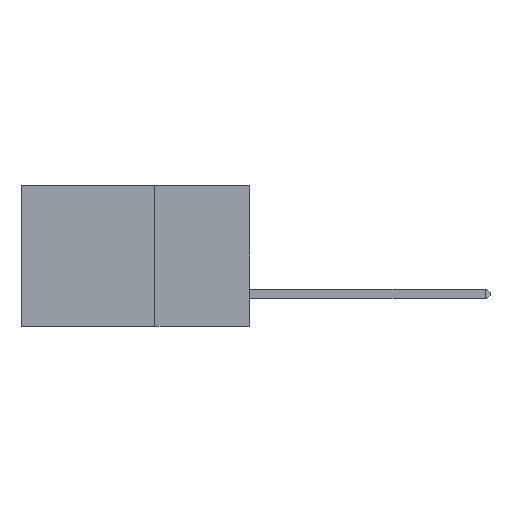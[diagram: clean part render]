
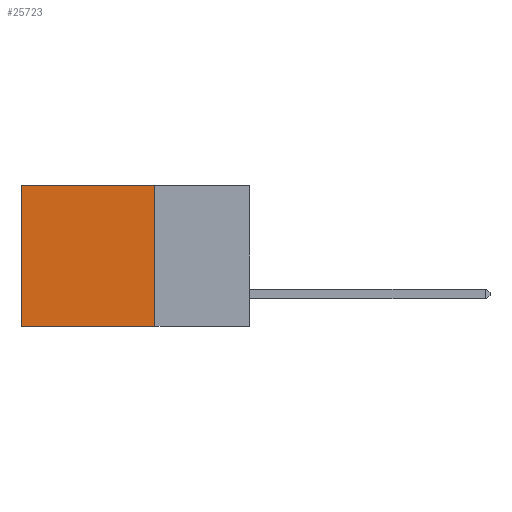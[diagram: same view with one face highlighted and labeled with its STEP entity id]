
A CAD part, left-side view. The second image highlights one B-rep face of the part: STEP entity #25723.
In plain terms, the highlighted planar face has unit normal (-1, 0, 0).
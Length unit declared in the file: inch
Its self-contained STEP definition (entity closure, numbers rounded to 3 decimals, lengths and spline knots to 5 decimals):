
#2175 = DIRECTION ( 'NONE',  ( 0., 1., 0. ) ) ;
#4576 = EDGE_CURVE ( 'NONE', #7238, #12971, #31821, .T. ) ;
#4618 = AXIS2_PLACEMENT_3D ( 'NONE', #30808, #13697, #33624 ) ;
#5003 = CARTESIAN_POINT ( 'NONE',  ( 0.2875, 0.25, -0.37 ) ) ;
#5343 = DIRECTION ( 'NONE',  ( 0., 0., -1. ) ) ;
#5471 = ORIENTED_EDGE ( 'NONE', *, *, #14323, .F. ) ;
#5676 = VECTOR ( 'NONE', #25467, 39.37008 ) ;
#6939 = LINE ( 'NONE', #13824, #34644 ) ;
#7238 = VERTEX_POINT ( 'NONE', #11531 ) ;
#8082 = CARTESIAN_POINT ( 'NONE',  ( 0.2875, 0.6, -0.37 ) ) ;
#8297 = CARTESIAN_POINT ( 'NONE',  ( 0.2875, 0.25, 0. ) ) ;
#10803 = PLANE ( 'NONE',  #4618 ) ;
#11531 = CARTESIAN_POINT ( 'NONE',  ( 0.2875, 0.25, 0. ) ) ;
#12971 = VERTEX_POINT ( 'NONE', #36786 ) ;
#13697 = DIRECTION ( 'NONE',  ( 1., 0., 0. ) ) ;
#13824 = CARTESIAN_POINT ( 'NONE',  ( 0.2875, 0.6, 0. ) ) ;
#14102 = CARTESIAN_POINT ( 'NONE',  ( 0.2875, 0.25, 0. ) ) ;
#14323 = EDGE_CURVE ( 'NONE', #7238, #36456, #36059, .T. ) ;
#21843 = ORIENTED_EDGE ( 'NONE', *, *, #23921, .T. ) ;
#23921 = EDGE_CURVE ( 'NONE', #12971, #34577, #6939, .T. ) ;
#25449 = DIRECTION ( 'NONE',  ( 0., 1., 0. ) ) ;
#25467 = DIRECTION ( 'NONE',  ( 0., 0., -1. ) ) ;
#25723 = ADVANCED_FACE ( 'NONE', ( #31357 ), #10803, .F. ) ;
#27373 = VECTOR ( 'NONE', #2175, 39.37008 ) ;
#27978 = ORIENTED_EDGE ( 'NONE', *, *, #4576, .T. ) ;
#29162 = LINE ( 'NONE', #5003, #27373 ) ;
#30808 = CARTESIAN_POINT ( 'NONE',  ( 0.2875, 0.25, 0. ) ) ;
#30893 = CARTESIAN_POINT ( 'NONE',  ( 0.2875, 0.25, -0.37 ) ) ;
#30956 = VECTOR ( 'NONE', #25449, 39.37008 ) ;
#31357 = FACE_OUTER_BOUND ( 'NONE', #32447, .T. ) ;
#31733 = ORIENTED_EDGE ( 'NONE', *, *, #32331, .F. ) ;
#31821 = LINE ( 'NONE', #8297, #30956 ) ;
#32331 = EDGE_CURVE ( 'NONE', #36456, #34577, #29162, .T. ) ;
#32447 = EDGE_LOOP ( 'NONE', ( #21843, #31733, #5471, #27978 ) ) ;
#33624 = DIRECTION ( 'NONE',  ( 0., 0., -1. ) ) ;
#34577 = VERTEX_POINT ( 'NONE', #8082 ) ;
#34644 = VECTOR ( 'NONE', #5343, 39.37008 ) ;
#36059 = LINE ( 'NONE', #14102, #5676 ) ;
#36456 = VERTEX_POINT ( 'NONE', #30893 ) ;
#36786 = CARTESIAN_POINT ( 'NONE',  ( 0.2875, 0.6, 0. ) ) ;
